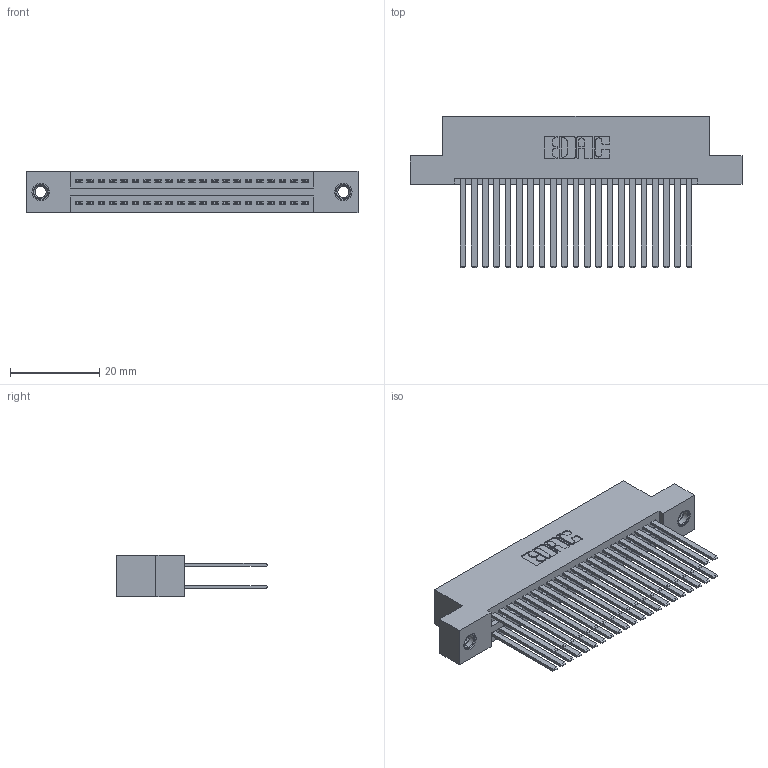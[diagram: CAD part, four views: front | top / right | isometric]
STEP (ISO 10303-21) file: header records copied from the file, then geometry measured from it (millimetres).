
FILE_DESCRIPTION (( 'STEP AP203' ), '1' );
FILE_NAME ('345-042-544-207.STEP', '2019-10-28T20:34:55', ( '' ), ( '' ), 'SwSTEP 2.0', 'SolidWorks 2016', '' );
FILE_SCHEMA (( 'CONFIG_CONTROL_DESIGN' ));
Length unit declared in the file: inch
Products named in the file (4): 345-042-544-207; 345 Part_Flush Mounting Lugs - 0.156 Dia-TI; 345-292-001_345-293-144; 345-250-001_345-250-005-103
Assembly tree (45 placements, depth 2):
  345-042-544-207
    345 Part_Flush Mounting Lugs - 0.156 Dia-TI
    345-292-001_345-293-144  x42
    345-250-001_345-250-005-103  x2
Bounding box: 74.55 x 33.96 x 9.4 mm (x, y, z)
Volume: 7622.1 mm3; surface area: 12613.5 mm2
Topology: 45 solids, 45 shells, 2034 faces, 5979 edges, 3922 vertices
Faces by surface type: plane 1330, cylinder 688, cone 12, torus 4
Entity records: 20306 total; most frequent: CARTESIAN_POINT 3403, ORIENTED_EDGE 3330, DIRECTION 3051, EDGE_CURVE 1665, VECTOR 1433, LINE 1433, VERTEX_POINT 1104, AXIS2_PLACEMENT_3D 809
